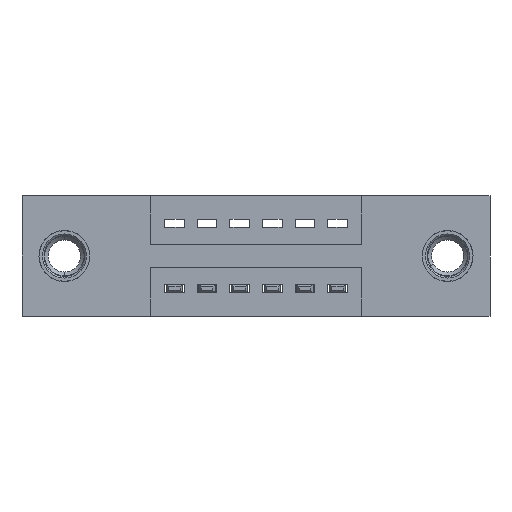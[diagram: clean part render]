
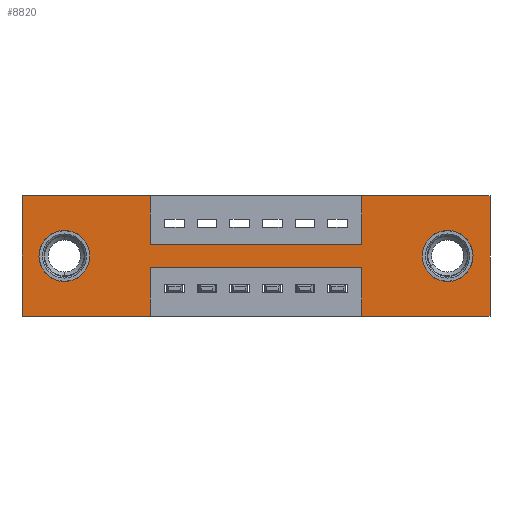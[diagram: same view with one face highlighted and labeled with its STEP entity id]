
A CAD part, front view. The second image highlights one B-rep face of the part: STEP entity #8820.
In plain terms, the highlighted planar face has unit normal (0, -1, 0).
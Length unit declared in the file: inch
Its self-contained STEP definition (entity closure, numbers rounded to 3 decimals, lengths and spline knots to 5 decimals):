
#12 = ORIENTED_EDGE ( 'NONE', *, *, #1825, .F. ) ;
#23 = ORIENTED_EDGE ( 'NONE', *, *, #4867, .T. ) ;
#24 = EDGE_LOOP ( 'NONE', ( #23, #838 ) ) ;
#31 = CARTESIAN_POINT ( 'NONE',  ( 0.13, 0., -0.263 ) ) ;
#57 = DIRECTION ( 'NONE',  ( 0., 1., 0. ) ) ;
#165 = VECTOR ( 'NONE', #4663, 39.37008 ) ;
#367 = EDGE_CURVE ( 'NONE', #7340, #1245, #2825, .T. ) ;
#376 = VECTOR ( 'NONE', #6025, 39.37008 ) ;
#547 = EDGE_CURVE ( 'NONE', #6975, #5453, #578, .T. ) ;
#573 = EDGE_CURVE ( 'NONE', #9424, #977, #4546, .T. ) ;
#578 = LINE ( 'NONE', #2548, #1684 ) ;
#579 = AXIS2_PLACEMENT_3D ( 'NONE', #8776, #57, #3961 ) ;
#656 = EDGE_CURVE ( 'NONE', #8329, #10175, #1436, .T. ) ;
#685 = CIRCLE ( 'NONE', #7212, 0.078 ) ;
#838 = ORIENTED_EDGE ( 'NONE', *, *, #2874, .T. ) ;
#877 = CARTESIAN_POINT ( 'NONE',  ( 0.3925, 0., -0.22 ) ) ;
#977 = VERTEX_POINT ( 'NONE', #1179 ) ;
#1010 = ORIENTED_EDGE ( 'NONE', *, *, #5736, .F. ) ;
#1080 = ORIENTED_EDGE ( 'NONE', *, *, #4517, .T. ) ;
#1179 = CARTESIAN_POINT ( 'NONE',  ( 0.3925, 0., 0. ) ) ;
#1245 = VERTEX_POINT ( 'NONE', #6050 ) ;
#1367 = ORIENTED_EDGE ( 'NONE', *, *, #6371, .F. ) ;
#1436 = LINE ( 'NONE', #3305, #7571 ) ;
#1568 = EDGE_CURVE ( 'NONE', #6075, #5408, #4018, .T. ) ;
#1684 = VECTOR ( 'NONE', #9762, 39.37008 ) ;
#1741 = VERTEX_POINT ( 'NONE', #9996 ) ;
#1745 = CARTESIAN_POINT ( 'NONE',  ( 0.13, 0., -0.185 ) ) ;
#1825 = EDGE_CURVE ( 'NONE', #977, #7514, #1913, .T. ) ;
#1913 = LINE ( 'NONE', #7938, #10184 ) ;
#2163 = LINE ( 'NONE', #5319, #6163 ) ;
#2266 = VERTEX_POINT ( 'NONE', #2836 ) ;
#2374 = CARTESIAN_POINT ( 'NONE',  ( 0.3925, 0., -0.22 ) ) ;
#2487 = VECTOR ( 'NONE', #8259, 39.37008 ) ;
#2514 = DIRECTION ( 'NONE',  ( 1., 0., 0. ) ) ;
#2548 = CARTESIAN_POINT ( 'NONE',  ( 0., 0., -0.37 ) ) ;
#2556 = DIRECTION ( 'NONE',  ( 0., 0., -1. ) ) ;
#2584 = DIRECTION ( 'NONE',  ( 0., 0., -1. ) ) ;
#2591 = CARTESIAN_POINT ( 'NONE',  ( 1.305, 0., -0.185 ) ) ;
#2677 = LINE ( 'NONE', #5416, #165 ) ;
#2688 = CARTESIAN_POINT ( 'NONE',  ( 1.435, 0., 0. ) ) ;
#2711 = CARTESIAN_POINT ( 'NONE',  ( 0., 0., -0.37 ) ) ;
#2731 = VERTEX_POINT ( 'NONE', #31 ) ;
#2825 = LINE ( 'NONE', #6367, #4298 ) ;
#2836 = CARTESIAN_POINT ( 'NONE',  ( 1.305, 0., -0.263 ) ) ;
#2846 = CARTESIAN_POINT ( 'NONE',  ( 0.3925, 0., -0.37 ) ) ;
#2874 = EDGE_CURVE ( 'NONE', #2731, #1741, #4361, .T. ) ;
#2884 = ORIENTED_EDGE ( 'NONE', *, *, #5365, .F. ) ;
#2925 = CARTESIAN_POINT ( 'NONE',  ( 0., 0., -0.37 ) ) ;
#2942 = EDGE_CURVE ( 'NONE', #4846, #6075, #3351, .T. ) ;
#3105 = DIRECTION ( 'NONE',  ( 0., 0., 1. ) ) ;
#3119 = AXIS2_PLACEMENT_3D ( 'NONE', #2711, #5772, #6632 ) ;
#3241 = CARTESIAN_POINT ( 'NONE',  ( 1.305, 0., -0.185 ) ) ;
#3260 = EDGE_CURVE ( 'NONE', #7514, #7340, #9633, .T. ) ;
#3268 = DIRECTION ( 'NONE',  ( 0., 0., -1. ) ) ;
#3293 = CARTESIAN_POINT ( 'NONE',  ( 1.0425, 0., -0.37 ) ) ;
#3305 = CARTESIAN_POINT ( 'NONE',  ( 1.435, 0., 0. ) ) ;
#3351 = LINE ( 'NONE', #3929, #7018 ) ;
#3488 = DIRECTION ( 'NONE',  ( 0., 1., 0. ) ) ;
#3500 = DIRECTION ( 'NONE',  ( 0., 1., 0. ) ) ;
#3715 = CARTESIAN_POINT ( 'NONE',  ( 0., 0., 0. ) ) ;
#3927 = ORIENTED_EDGE ( 'NONE', *, *, #7568, .F. ) ;
#3929 = CARTESIAN_POINT ( 'NONE',  ( 1.0425, 0., -0.37 ) ) ;
#3956 = CARTESIAN_POINT ( 'NONE',  ( 1.435, 0., -0.37 ) ) ;
#3961 = DIRECTION ( 'NONE',  ( 0., 0., 1. ) ) ;
#3974 = DIRECTION ( 'NONE',  ( 0., 0., -1. ) ) ;
#4018 = LINE ( 'NONE', #2374, #9173 ) ;
#4028 = CARTESIAN_POINT ( 'NONE',  ( 0., 0., -0.37 ) ) ;
#4096 = CARTESIAN_POINT ( 'NONE',  ( 1.0425, 0., -0.15 ) ) ;
#4240 = DIRECTION ( 'NONE',  ( 0., 0., 1. ) ) ;
#4285 = AXIS2_PLACEMENT_3D ( 'NONE', #1745, #3488, #4240 ) ;
#4298 = VECTOR ( 'NONE', #3105, 39.37008 ) ;
#4361 = CIRCLE ( 'NONE', #4285, 0.078 ) ;
#4517 = EDGE_CURVE ( 'NONE', #2266, #10212, #685, .T. ) ;
#4546 = LINE ( 'NONE', #7318, #5164 ) ;
#4571 = EDGE_LOOP ( 'NONE', ( #1010, #9121, #9410, #1367, #8383, #3927, #7349, #9708, #12, #8950, #2884, #6278 ) ) ;
#4663 = DIRECTION ( 'NONE',  ( 0., 0., 1. ) ) ;
#4666 = CIRCLE ( 'NONE', #10225, 0.078 ) ;
#4705 = FACE_OUTER_BOUND ( 'NONE', #4571, .T. ) ;
#4846 = VERTEX_POINT ( 'NONE', #3293 ) ;
#4867 = EDGE_CURVE ( 'NONE', #1741, #2731, #9438, .T. ) ;
#4909 = DIRECTION ( 'NONE',  ( 0., 1., 0. ) ) ;
#5098 = CARTESIAN_POINT ( 'NONE',  ( 1.0425, 0., -0.22 ) ) ;
#5164 = VECTOR ( 'NONE', #2514, 39.37008 ) ;
#5201 = EDGE_CURVE ( 'NONE', #10212, #2266, #4666, .T. ) ;
#5319 = CARTESIAN_POINT ( 'NONE',  ( 0.3925, 0., -0.37 ) ) ;
#5365 = EDGE_CURVE ( 'NONE', #5453, #9424, #2677, .T. ) ;
#5408 = VERTEX_POINT ( 'NONE', #877 ) ;
#5416 = CARTESIAN_POINT ( 'NONE',  ( 0., 0., 0. ) ) ;
#5453 = VERTEX_POINT ( 'NONE', #4028 ) ;
#5538 = DIRECTION ( 'NONE',  ( -1., 0., 0. ) ) ;
#5717 = LINE ( 'NONE', #3715, #376 ) ;
#5736 = EDGE_CURVE ( 'NONE', #5408, #6975, #2163, .T. ) ;
#5772 = DIRECTION ( 'NONE',  ( 0., -1., 0. ) ) ;
#5806 = CARTESIAN_POINT ( 'NONE',  ( 0.3925, 0., -0.15 ) ) ;
#5866 = CARTESIAN_POINT ( 'NONE',  ( 0.3925, 0., -0.15 ) ) ;
#6004 = CARTESIAN_POINT ( 'NONE',  ( 1.305, 0., -0.107 ) ) ;
#6016 = VECTOR ( 'NONE', #8516, 39.37008 ) ;
#6025 = DIRECTION ( 'NONE',  ( 1., 0., 0. ) ) ;
#6050 = CARTESIAN_POINT ( 'NONE',  ( 1.0425, 0., 0. ) ) ;
#6075 = VERTEX_POINT ( 'NONE', #5098 ) ;
#6126 = DIRECTION ( 'NONE',  ( 0., 0., -1. ) ) ;
#6163 = VECTOR ( 'NONE', #6126, 39.37008 ) ;
#6278 = ORIENTED_EDGE ( 'NONE', *, *, #547, .F. ) ;
#6344 = FACE_BOUND ( 'NONE', #8526, .T. ) ;
#6367 = CARTESIAN_POINT ( 'NONE',  ( 1.0425, 0., 0. ) ) ;
#6371 = EDGE_CURVE ( 'NONE', #10175, #4846, #7903, .T. ) ;
#6632 = DIRECTION ( 'NONE',  ( 0., 0., -1. ) ) ;
#6668 = PLANE ( 'NONE',  #3119 ) ;
#6975 = VERTEX_POINT ( 'NONE', #2846 ) ;
#7018 = VECTOR ( 'NONE', #7900, 39.37008 ) ;
#7212 = AXIS2_PLACEMENT_3D ( 'NONE', #2591, #3500, #2556 ) ;
#7318 = CARTESIAN_POINT ( 'NONE',  ( 0., 0., 0. ) ) ;
#7340 = VERTEX_POINT ( 'NONE', #4096 ) ;
#7349 = ORIENTED_EDGE ( 'NONE', *, *, #367, .F. ) ;
#7514 = VERTEX_POINT ( 'NONE', #5806 ) ;
#7568 = EDGE_CURVE ( 'NONE', #1245, #8329, #5717, .T. ) ;
#7571 = VECTOR ( 'NONE', #3268, 39.37008 ) ;
#7611 = FACE_BOUND ( 'NONE', #24, .T. ) ;
#7900 = DIRECTION ( 'NONE',  ( 0., 0., 1. ) ) ;
#7903 = LINE ( 'NONE', #2925, #6016 ) ;
#7938 = CARTESIAN_POINT ( 'NONE',  ( 0.3925, 0., 0. ) ) ;
#8072 = CARTESIAN_POINT ( 'NONE',  ( 0., 0., 0. ) ) ;
#8259 = DIRECTION ( 'NONE',  ( 1., 0., 0. ) ) ;
#8329 = VERTEX_POINT ( 'NONE', #2688 ) ;
#8383 = ORIENTED_EDGE ( 'NONE', *, *, #656, .F. ) ;
#8516 = DIRECTION ( 'NONE',  ( -1., 0., 0. ) ) ;
#8526 = EDGE_LOOP ( 'NONE', ( #8614, #1080 ) ) ;
#8614 = ORIENTED_EDGE ( 'NONE', *, *, #5201, .T. ) ;
#8776 = CARTESIAN_POINT ( 'NONE',  ( 0.13, 0., -0.185 ) ) ;
#8820 = ADVANCED_FACE ( 'NONE', ( #6344, #7611, #4705 ), #6668, .T. ) ;
#8950 = ORIENTED_EDGE ( 'NONE', *, *, #573, .F. ) ;
#9121 = ORIENTED_EDGE ( 'NONE', *, *, #1568, .F. ) ;
#9173 = VECTOR ( 'NONE', #5538, 39.37008 ) ;
#9410 = ORIENTED_EDGE ( 'NONE', *, *, #2942, .F. ) ;
#9424 = VERTEX_POINT ( 'NONE', #8072 ) ;
#9438 = CIRCLE ( 'NONE', #579, 0.078 ) ;
#9633 = LINE ( 'NONE', #5866, #2487 ) ;
#9708 = ORIENTED_EDGE ( 'NONE', *, *, #3260, .F. ) ;
#9762 = DIRECTION ( 'NONE',  ( -1., 0., 0. ) ) ;
#9996 = CARTESIAN_POINT ( 'NONE',  ( 0.13, 0., -0.107 ) ) ;
#10175 = VERTEX_POINT ( 'NONE', #3956 ) ;
#10184 = VECTOR ( 'NONE', #3974, 39.37008 ) ;
#10212 = VERTEX_POINT ( 'NONE', #6004 ) ;
#10225 = AXIS2_PLACEMENT_3D ( 'NONE', #3241, #4909, #2584 ) ;
